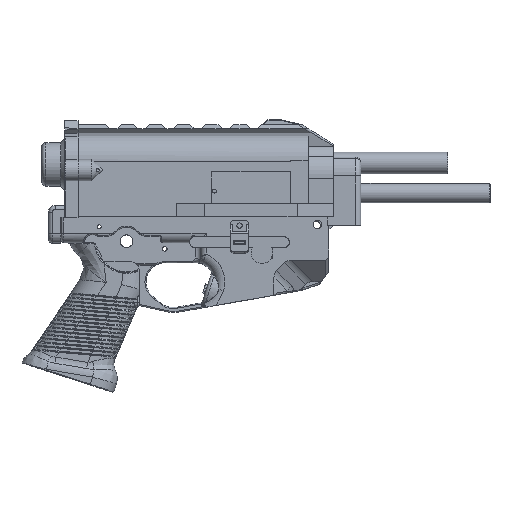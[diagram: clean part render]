
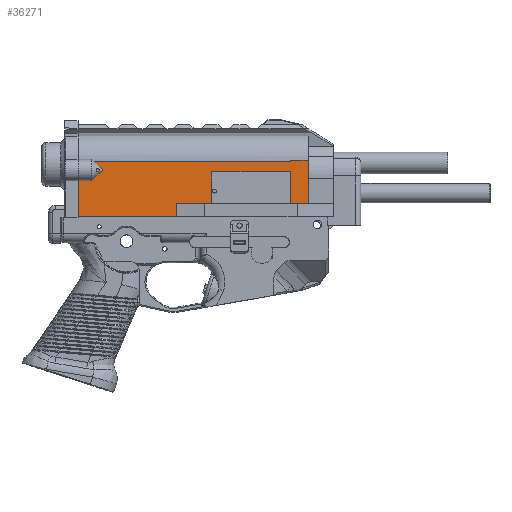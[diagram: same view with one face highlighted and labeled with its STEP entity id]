
A CAD part, top view. The second image highlights one B-rep face of the part: STEP entity #36271.
In plain terms, the highlighted planar face has unit normal (0, 0, 1).
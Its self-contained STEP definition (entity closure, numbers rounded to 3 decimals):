
#2893=PLANE('',#38818);
#4195=FACE_OUTER_BOUND('',#6295,.T.);
#6295=EDGE_LOOP('',(#27250,#27251,#27252,#27253,#27254,#27255,#27256,#27257,
#27258,#27259,#27260,#27261,#27262,#27263,#27264,#27265));
#9778=LINE('',#53469,#13259);
#9852=LINE('',#53649,#13333);
#9854=LINE('',#53653,#13335);
#9856=LINE('',#53657,#13337);
#9858=LINE('',#53661,#13339);
#9865=LINE('',#53674,#13346);
#10021=LINE('',#54044,#13502);
#10033=LINE('',#54066,#13514);
#10034=LINE('',#54068,#13515);
#10035=LINE('',#54070,#13516);
#10036=LINE('',#54072,#13517);
#10037=LINE('',#54074,#13518);
#10038=LINE('',#54076,#13519);
#10039=LINE('',#54078,#13520);
#10040=LINE('',#54079,#13521);
#10041=LINE('',#54080,#13522);
#13259=VECTOR('',#43141,1.);
#13333=VECTOR('',#43279,1.);
#13335=VECTOR('',#43283,1.);
#13337=VECTOR('',#43287,1.);
#13339=VECTOR('',#43291,1.);
#13346=VECTOR('',#43298,1.);
#13502=VECTOR('',#43650,1.);
#13514=VECTOR('',#43664,1.);
#13515=VECTOR('',#43665,1.);
#13516=VECTOR('',#43666,1.);
#13517=VECTOR('',#43667,1.);
#13518=VECTOR('',#43668,1.);
#13519=VECTOR('',#43669,1.);
#13520=VECTOR('',#43670,1.);
#13521=VECTOR('',#43671,1.);
#13522=VECTOR('',#43672,1.);
#16582=VERTEX_POINT('',#53466);
#16583=VERTEX_POINT('',#53468);
#16648=VERTEX_POINT('',#53646);
#16649=VERTEX_POINT('',#53648);
#16650=VERTEX_POINT('',#53652);
#16651=VERTEX_POINT('',#53656);
#16652=VERTEX_POINT('',#53660);
#16658=VERTEX_POINT('',#53672);
#16774=VERTEX_POINT('',#54042);
#16783=VERTEX_POINT('',#54065);
#16784=VERTEX_POINT('',#54067);
#16785=VERTEX_POINT('',#54069);
#16786=VERTEX_POINT('',#54071);
#16787=VERTEX_POINT('',#54073);
#16788=VERTEX_POINT('',#54075);
#16789=VERTEX_POINT('',#54077);
#20396=EDGE_CURVE('',#16583,#16582,#9778,.T.);
#20486=EDGE_CURVE('',#16649,#16648,#9852,.T.);
#20488=EDGE_CURVE('',#16650,#16649,#9854,.T.);
#20490=EDGE_CURVE('',#16651,#16650,#9856,.T.);
#20492=EDGE_CURVE('',#16652,#16651,#9858,.T.);
#20499=EDGE_CURVE('',#16648,#16658,#9865,.T.);
#20686=EDGE_CURVE('',#16774,#16582,#10021,.T.);
#20698=EDGE_CURVE('',#16658,#16783,#10033,.T.);
#20699=EDGE_CURVE('',#16783,#16784,#10034,.T.);
#20700=EDGE_CURVE('',#16784,#16785,#10035,.T.);
#20701=EDGE_CURVE('',#16785,#16786,#10036,.T.);
#20702=EDGE_CURVE('',#16786,#16787,#10037,.T.);
#20703=EDGE_CURVE('',#16787,#16788,#10038,.T.);
#20704=EDGE_CURVE('',#16788,#16789,#10039,.T.);
#20705=EDGE_CURVE('',#16789,#16583,#10040,.T.);
#20706=EDGE_CURVE('',#16774,#16652,#10041,.T.);
#27250=ORIENTED_EDGE('',*,*,#20492,.T.);
#27251=ORIENTED_EDGE('',*,*,#20490,.T.);
#27252=ORIENTED_EDGE('',*,*,#20488,.T.);
#27253=ORIENTED_EDGE('',*,*,#20486,.T.);
#27254=ORIENTED_EDGE('',*,*,#20499,.T.);
#27255=ORIENTED_EDGE('',*,*,#20698,.T.);
#27256=ORIENTED_EDGE('',*,*,#20699,.T.);
#27257=ORIENTED_EDGE('',*,*,#20700,.T.);
#27258=ORIENTED_EDGE('',*,*,#20701,.T.);
#27259=ORIENTED_EDGE('',*,*,#20702,.T.);
#27260=ORIENTED_EDGE('',*,*,#20703,.T.);
#27261=ORIENTED_EDGE('',*,*,#20704,.T.);
#27262=ORIENTED_EDGE('',*,*,#20705,.T.);
#27263=ORIENTED_EDGE('',*,*,#20396,.T.);
#27264=ORIENTED_EDGE('',*,*,#20686,.F.);
#27265=ORIENTED_EDGE('',*,*,#20706,.T.);
#36271=ADVANCED_FACE('',(#4195),#2893,.T.);
#38818=AXIS2_PLACEMENT_3D('',#54064,#43662,#43663);
#43141=DIRECTION('',(0.,-1.,0.));
#43279=DIRECTION('',(0.,-1.,0.));
#43283=DIRECTION('',(1.,0.,0.));
#43287=DIRECTION('',(0.,1.,0.));
#43291=DIRECTION('',(1.,0.,0.));
#43298=DIRECTION('',(1.,0.,0.));
#43650=DIRECTION('',(-1.,0.,0.));
#43662=DIRECTION('center_axis',(0.,0.,1.));
#43663=DIRECTION('ref_axis',(1.,0.,0.));
#43664=DIRECTION('',(0.,1.,0.));
#43665=DIRECTION('',(-1.,0.,0.));
#43666=DIRECTION('',(0.,-1.,0.));
#43667=DIRECTION('',(-1.,0.,0.));
#43668=DIRECTION('',(0.707,-0.707,0.));
#43669=DIRECTION('',(0.,-1.,0.));
#43670=DIRECTION('',(-0.707,-0.707,0.));
#43671=DIRECTION('',(-1.,0.,0.));
#43672=DIRECTION('',(0.,1.,0.));
#53466=CARTESIAN_POINT('',(-178.497,6.49,20.1));
#53468=CARTESIAN_POINT('',(-178.497,33.428,20.1));
#53469=CARTESIAN_POINT('',(-178.497,48.04,20.1));
#53646=CARTESIAN_POINT('',(-19.97,16.49,20.1));
#53648=CARTESIAN_POINT('',(-19.97,40.076,20.1));
#53649=CARTESIAN_POINT('',(-19.97,48.04,20.1));
#53652=CARTESIAN_POINT('',(-78.815,40.076,20.1));
#53653=CARTESIAN_POINT('',(-19.865,40.076,20.1));
#53656=CARTESIAN_POINT('',(-78.815,16.49,20.1));
#53657=CARTESIAN_POINT('',(-78.815,48.04,20.1));
#53660=CARTESIAN_POINT('',(-105.221,16.49,20.1));
#53661=CARTESIAN_POINT('',(-19.865,16.49,20.1));
#53672=CARTESIAN_POINT('',(-6.865,16.49,20.1));
#53674=CARTESIAN_POINT('',(-19.865,16.49,20.1));
#54042=CARTESIAN_POINT('',(-105.221,6.49,20.1));
#54044=CARTESIAN_POINT('',(-159.565,6.49,20.1));
#54064=CARTESIAN_POINT('Origin',(-19.865,48.04,20.1));
#54065=CARTESIAN_POINT('',(-6.865,48.66,20.1));
#54066=CARTESIAN_POINT('',(-6.865,-4.94,20.1));
#54067=CARTESIAN_POINT('',(-19.865,48.66,20.1));
#54068=CARTESIAN_POINT('',(-2.359,48.66,20.1));
#54069=CARTESIAN_POINT('',(-19.865,48.04,20.1));
#54070=CARTESIAN_POINT('',(-19.865,-4.94,20.1));
#54071=CARTESIAN_POINT('',(-166.91,48.04,20.1));
#54072=CARTESIAN_POINT('',(-19.865,48.04,20.1));
#54073=CARTESIAN_POINT('',(-160.497,41.628,20.1));
#54074=CARTESIAN_POINT('',(-166.91,48.04,20.1));
#54075=CARTESIAN_POINT('',(-160.497,41.228,20.1));
#54076=CARTESIAN_POINT('',(-160.497,48.04,20.1));
#54077=CARTESIAN_POINT('',(-168.297,33.428,20.1));
#54078=CARTESIAN_POINT('',(-160.497,41.228,20.1));
#54079=CARTESIAN_POINT('',(-19.865,33.428,20.1));
#54080=CARTESIAN_POINT('',(-105.221,48.04,20.1));
